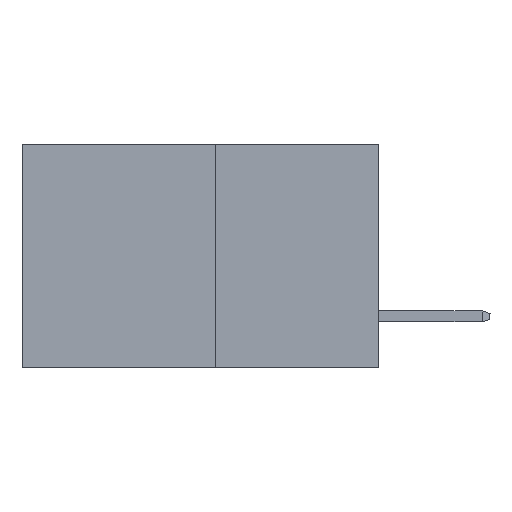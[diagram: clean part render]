
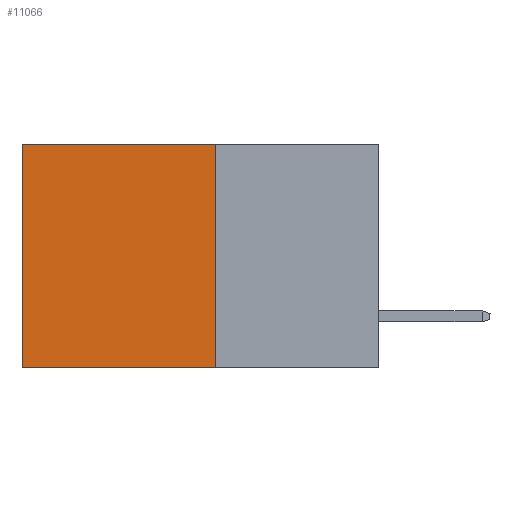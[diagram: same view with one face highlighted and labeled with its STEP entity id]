
A CAD part, left-side view. The second image highlights one B-rep face of the part: STEP entity #11066.
In plain terms, the highlighted planar face has unit normal (-1, 0, 0).
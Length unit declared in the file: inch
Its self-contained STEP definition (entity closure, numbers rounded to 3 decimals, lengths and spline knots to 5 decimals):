
#664 = CARTESIAN_POINT ( 'NONE',  ( 0.277, 0.27, 0. ) ) ;
#1073 = VERTEX_POINT ( 'NONE', #1478 ) ;
#1308 = DIRECTION ( 'NONE',  ( 0., 0., -1. ) ) ;
#1478 = CARTESIAN_POINT ( 'NONE',  ( 0.277, 0.59, 0. ) ) ;
#2446 = DIRECTION ( 'NONE',  ( 0., 1., 0. ) ) ;
#2465 = VECTOR ( 'NONE', #3085, 39.37008 ) ;
#2655 = VECTOR ( 'NONE', #14517, 39.37008 ) ;
#2666 = EDGE_CURVE ( 'NONE', #9252, #10717, #6709, .T. ) ;
#3085 = DIRECTION ( 'NONE',  ( 0., 1., 0. ) ) ;
#3283 = EDGE_CURVE ( 'NONE', #1073, #15563, #5922, .T. ) ;
#3633 = VECTOR ( 'NONE', #2446, 39.37008 ) ;
#3776 = EDGE_LOOP ( 'NONE', ( #14185, #9077, #12070, #7528 ) ) ;
#4802 = DIRECTION ( 'NONE',  ( 1., 0., 0. ) ) ;
#5168 = EDGE_CURVE ( 'NONE', #9252, #1073, #9828, .T. ) ;
#5922 = LINE ( 'NONE', #14278, #2655 ) ;
#6222 = FACE_OUTER_BOUND ( 'NONE', #3776, .T. ) ;
#6709 = LINE ( 'NONE', #7150, #9625 ) ;
#6761 = EDGE_CURVE ( 'NONE', #10717, #15563, #12375, .T. ) ;
#7150 = CARTESIAN_POINT ( 'NONE',  ( 0.277, 0.27, -0.37 ) ) ;
#7528 = ORIENTED_EDGE ( 'NONE', *, *, #5168, .T. ) ;
#8480 = PLANE ( 'NONE',  #9407 ) ;
#9077 = ORIENTED_EDGE ( 'NONE', *, *, #6761, .F. ) ;
#9252 = VERTEX_POINT ( 'NONE', #664 ) ;
#9407 = AXIS2_PLACEMENT_3D ( 'NONE', #12302, #4802, #13547 ) ;
#9557 = CARTESIAN_POINT ( 'NONE',  ( 0.277, 0.27, -0.37 ) ) ;
#9625 = VECTOR ( 'NONE', #1308, 39.37008 ) ;
#9828 = LINE ( 'NONE', #9833, #3633 ) ;
#9833 = CARTESIAN_POINT ( 'NONE',  ( 0.277, 0.27, 0. ) ) ;
#10717 = VERTEX_POINT ( 'NONE', #9557 ) ;
#11066 = ADVANCED_FACE ( 'NONE', ( #6222 ), #8480, .F. ) ;
#12070 = ORIENTED_EDGE ( 'NONE', *, *, #2666, .F. ) ;
#12302 = CARTESIAN_POINT ( 'NONE',  ( 0.277, 0.27, -0.37 ) ) ;
#12320 = CARTESIAN_POINT ( 'NONE',  ( 0.277, 0.59, -0.37 ) ) ;
#12375 = LINE ( 'NONE', #14234, #2465 ) ;
#13547 = DIRECTION ( 'NONE',  ( 0., 0., -1. ) ) ;
#14185 = ORIENTED_EDGE ( 'NONE', *, *, #3283, .T. ) ;
#14234 = CARTESIAN_POINT ( 'NONE',  ( 0.277, 0.27, -0.37 ) ) ;
#14278 = CARTESIAN_POINT ( 'NONE',  ( 0.277, 0.59, -0.37 ) ) ;
#14517 = DIRECTION ( 'NONE',  ( 0., 0., -1. ) ) ;
#15563 = VERTEX_POINT ( 'NONE', #12320 ) ;
